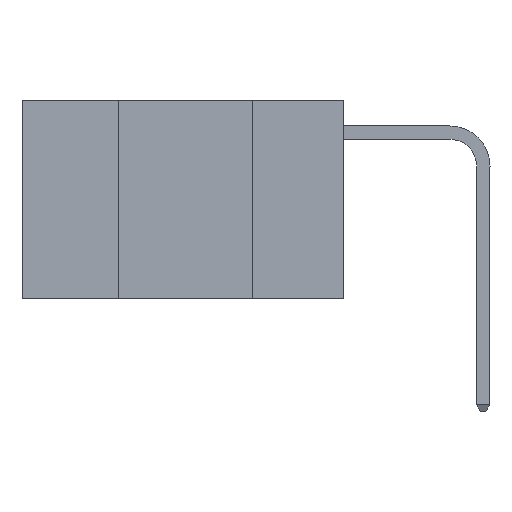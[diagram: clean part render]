
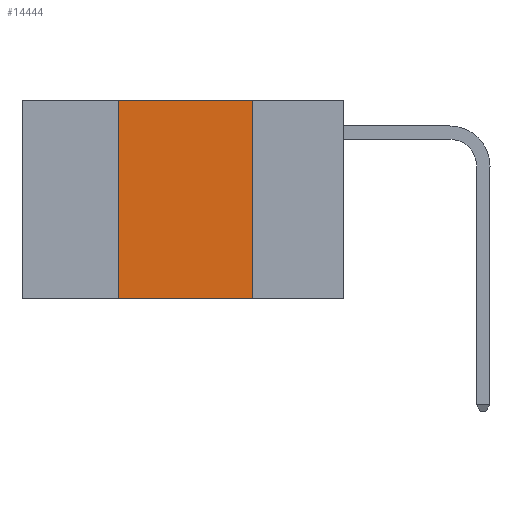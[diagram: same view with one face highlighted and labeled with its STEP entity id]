
A CAD part, left-side view. The second image highlights one B-rep face of the part: STEP entity #14444.
In plain terms, the highlighted planar face has unit normal (-1, 0, 0).
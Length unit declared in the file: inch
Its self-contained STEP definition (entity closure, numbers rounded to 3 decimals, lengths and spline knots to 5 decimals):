
#1057 = VERTEX_POINT ( 'NONE', #7448 ) ;
#1151 = LINE ( 'NONE', #10103, #4548 ) ;
#1341 = EDGE_CURVE ( 'NONE', #3120, #1057, #5013, .T. ) ;
#2337 = VERTEX_POINT ( 'NONE', #14296 ) ;
#3032 = VECTOR ( 'NONE', #13282, 39.37008 ) ;
#3120 = VERTEX_POINT ( 'NONE', #11823 ) ;
#3729 = EDGE_LOOP ( 'NONE', ( #11396, #11576, #11673, #11717 ) ) ;
#3740 = VECTOR ( 'NONE', #13051, 39.37008 ) ;
#4548 = VECTOR ( 'NONE', #13382, 39.37008 ) ;
#5013 = LINE ( 'NONE', #10319, #5072 ) ;
#5041 = CARTESIAN_POINT ( 'NONE',  ( 0., 0.17, -0.37 ) ) ;
#5072 = VECTOR ( 'NONE', #10269, 39.37008 ) ;
#5269 = EDGE_CURVE ( 'NONE', #2337, #12503, #8371, .T. ) ;
#6027 = EDGE_CURVE ( 'NONE', #2337, #3120, #1151, .T. ) ;
#6781 = EDGE_CURVE ( 'NONE', #1057, #12503, #9143, .T. ) ;
#6916 = PLANE ( 'NONE',  #8882 ) ;
#7448 = CARTESIAN_POINT ( 'NONE',  ( 0., 0.17, 0. ) ) ;
#8079 = DIRECTION ( 'NONE',  ( 0., 0., -1. ) ) ;
#8371 = LINE ( 'NONE', #13648, #3740 ) ;
#8634 = FACE_OUTER_BOUND ( 'NONE', #3729, .T. ) ;
#8882 = AXIS2_PLACEMENT_3D ( 'NONE', #11507, #14586, #8079 ) ;
#9143 = LINE ( 'NONE', #12258, #3032 ) ;
#10103 = CARTESIAN_POINT ( 'NONE',  ( 0., 0.42, 0. ) ) ;
#10269 = DIRECTION ( 'NONE',  ( 0., -1., 0. ) ) ;
#10319 = CARTESIAN_POINT ( 'NONE',  ( 0., 0.6, 0. ) ) ;
#11396 = ORIENTED_EDGE ( 'NONE', *, *, #6781, .F. ) ;
#11507 = CARTESIAN_POINT ( 'NONE',  ( 0., 0.6, 0. ) ) ;
#11576 = ORIENTED_EDGE ( 'NONE', *, *, #1341, .F. ) ;
#11673 = ORIENTED_EDGE ( 'NONE', *, *, #6027, .F. ) ;
#11717 = ORIENTED_EDGE ( 'NONE', *, *, #5269, .T. ) ;
#11823 = CARTESIAN_POINT ( 'NONE',  ( 0., 0.42, 0. ) ) ;
#12258 = CARTESIAN_POINT ( 'NONE',  ( 0., 0.17, 0. ) ) ;
#12503 = VERTEX_POINT ( 'NONE', #5041 ) ;
#13051 = DIRECTION ( 'NONE',  ( 0., -1., 0. ) ) ;
#13282 = DIRECTION ( 'NONE',  ( 0., 0., -1. ) ) ;
#13382 = DIRECTION ( 'NONE',  ( 0., 0., 1. ) ) ;
#13648 = CARTESIAN_POINT ( 'NONE',  ( 0., 0.6, -0.37 ) ) ;
#14296 = CARTESIAN_POINT ( 'NONE',  ( 0., 0.42, -0.37 ) ) ;
#14444 = ADVANCED_FACE ( 'NONE', ( #8634 ), #6916, .F. ) ;
#14586 = DIRECTION ( 'NONE',  ( 1., 0., 0. ) ) ;
